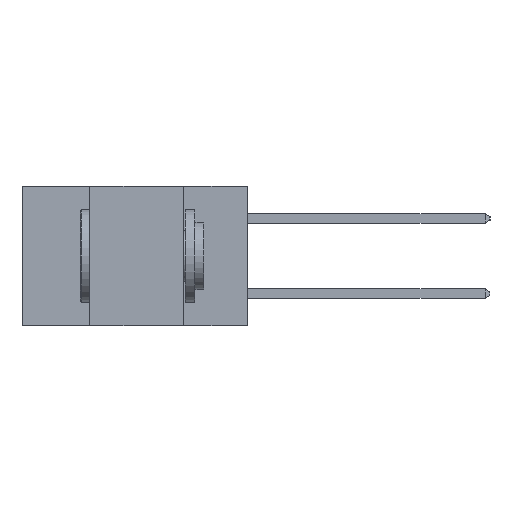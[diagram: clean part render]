
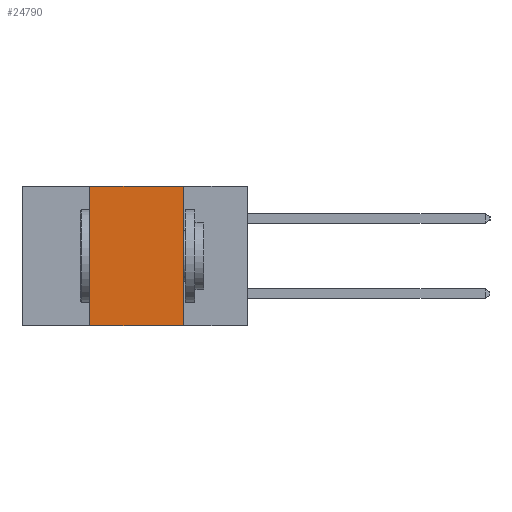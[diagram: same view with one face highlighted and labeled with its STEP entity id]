
A CAD part, left-side view. The second image highlights one B-rep face of the part: STEP entity #24790.
In plain terms, the highlighted planar face has unit normal (-1, 0, 0).
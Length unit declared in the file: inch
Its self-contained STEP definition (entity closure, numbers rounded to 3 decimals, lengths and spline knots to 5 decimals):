
#372 = VERTEX_POINT ( 'NONE', #15070 ) ;
#469 = FACE_OUTER_BOUND ( 'NONE', #21587, .T. ) ;
#2493 = EDGE_CURVE ( 'NONE', #6450, #26914, #23003, .T. ) ;
#5378 = CARTESIAN_POINT ( 'NONE',  ( 0., 0.42, 0. ) ) ;
#5421 = EDGE_CURVE ( 'NONE', #6450, #16628, #9100, .T. ) ;
#5787 = EDGE_CURVE ( 'NONE', #372, #26914, #24835, .T. ) ;
#6450 = VERTEX_POINT ( 'NONE', #17252 ) ;
#7294 = DIRECTION ( 'NONE',  ( 0., 0., 1. ) ) ;
#7891 = VECTOR ( 'NONE', #13158, 39.37008 ) ;
#8257 = VECTOR ( 'NONE', #25995, 39.37008 ) ;
#8994 = CARTESIAN_POINT ( 'NONE',  ( 0., 0.6, 0. ) ) ;
#9100 = LINE ( 'NONE', #17946, #16620 ) ;
#11302 = ORIENTED_EDGE ( 'NONE', *, *, #5787, .F. ) ;
#11615 = DIRECTION ( 'NONE',  ( 1., 0., 0. ) ) ;
#13158 = DIRECTION ( 'NONE',  ( 0., 0., -1. ) ) ;
#15046 = CARTESIAN_POINT ( 'NONE',  ( 0., 0.6, -0.37 ) ) ;
#15070 = CARTESIAN_POINT ( 'NONE',  ( 0., 0.17, 0. ) ) ;
#15315 = DIRECTION ( 'NONE',  ( 0., -1., 0. ) ) ;
#15618 = ORIENTED_EDGE ( 'NONE', *, *, #2493, .T. ) ;
#16620 = VECTOR ( 'NONE', #7294, 39.37008 ) ;
#16628 = VERTEX_POINT ( 'NONE', #5378 ) ;
#17252 = CARTESIAN_POINT ( 'NONE',  ( 0., 0.42, -0.37 ) ) ;
#17401 = VECTOR ( 'NONE', #15315, 39.37008 ) ;
#17946 = CARTESIAN_POINT ( 'NONE',  ( 0., 0.42, -0.37 ) ) ;
#18892 = EDGE_CURVE ( 'NONE', #16628, #372, #25175, .T. ) ;
#21587 = EDGE_LOOP ( 'NONE', ( #11302, #27525, #26859, #15618 ) ) ;
#22042 = PLANE ( 'NONE',  #24816 ) ;
#23003 = LINE ( 'NONE', #15046, #17401 ) ;
#23658 = CARTESIAN_POINT ( 'NONE',  ( 0., 0.17, -0.37 ) ) ;
#24253 = CARTESIAN_POINT ( 'NONE',  ( 0., 0.6, 0. ) ) ;
#24520 = CARTESIAN_POINT ( 'NONE',  ( 0., 0.17, -0.37 ) ) ;
#24790 = ADVANCED_FACE ( 'NONE', ( #469 ), #22042, .F. ) ;
#24816 = AXIS2_PLACEMENT_3D ( 'NONE', #24253, #11615, #26439 ) ;
#24835 = LINE ( 'NONE', #23658, #7891 ) ;
#25175 = LINE ( 'NONE', #8994, #8257 ) ;
#25995 = DIRECTION ( 'NONE',  ( 0., -1., 0. ) ) ;
#26439 = DIRECTION ( 'NONE',  ( 0., 0., -1. ) ) ;
#26859 = ORIENTED_EDGE ( 'NONE', *, *, #5421, .F. ) ;
#26914 = VERTEX_POINT ( 'NONE', #24520 ) ;
#27525 = ORIENTED_EDGE ( 'NONE', *, *, #18892, .F. ) ;
